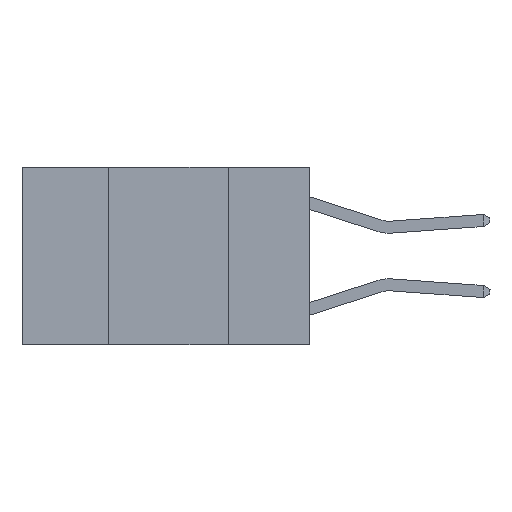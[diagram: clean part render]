
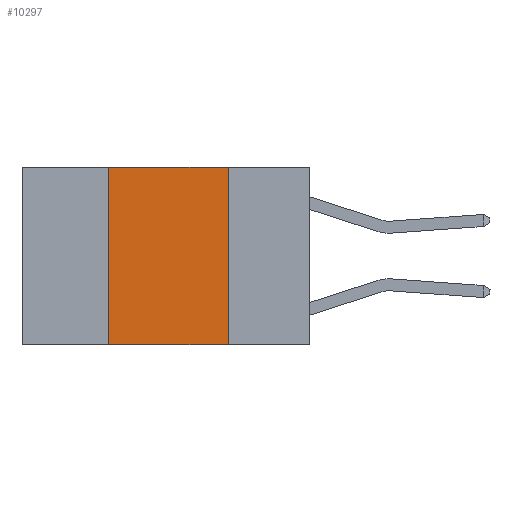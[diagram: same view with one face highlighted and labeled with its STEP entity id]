
A CAD part, left-side view. The second image highlights one B-rep face of the part: STEP entity #10297.
In plain terms, the highlighted planar face has unit normal (-1, 0, 0).
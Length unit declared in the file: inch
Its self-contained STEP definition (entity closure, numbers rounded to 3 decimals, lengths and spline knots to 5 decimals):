
#68 = DIRECTION ( 'NONE',  ( 0., 0., 1. ) ) ;
#74 = CARTESIAN_POINT ( 'NONE',  ( 0., 0.6, 0. ) ) ;
#545 = EDGE_CURVE ( 'NONE', #13243, #10573, #12109, .T. ) ;
#1654 = CARTESIAN_POINT ( 'NONE',  ( 0., 0.42, -0.37 ) ) ;
#2096 = LINE ( 'NONE', #6562, #13497 ) ;
#3424 = DIRECTION ( 'NONE',  ( 1., 0., 0. ) ) ;
#3793 = EDGE_CURVE ( 'NONE', #12015, #11036, #11168, .T. ) ;
#4370 = EDGE_CURVE ( 'NONE', #10573, #12015, #13056, .T. ) ;
#4399 = DIRECTION ( 'NONE',  ( 0., -1., 0. ) ) ;
#4626 = CARTESIAN_POINT ( 'NONE',  ( 0., 0.17, -0.37 ) ) ;
#4745 = FACE_OUTER_BOUND ( 'NONE', #12834, .T. ) ;
#5888 = VECTOR ( 'NONE', #68, 39.37008 ) ;
#6309 = CARTESIAN_POINT ( 'NONE',  ( 0., 0.17, 0. ) ) ;
#6562 = CARTESIAN_POINT ( 'NONE',  ( 0., 0.6, -0.37 ) ) ;
#7415 = DIRECTION ( 'NONE',  ( 0., 0., -1. ) ) ;
#7454 = ORIENTED_EDGE ( 'NONE', *, *, #4370, .F. ) ;
#7796 = ORIENTED_EDGE ( 'NONE', *, *, #12215, .T. ) ;
#8273 = DIRECTION ( 'NONE',  ( 0., -1., 0. ) ) ;
#8881 = CARTESIAN_POINT ( 'NONE',  ( 0., 0.42, 0. ) ) ;
#10297 = ADVANCED_FACE ( 'NONE', ( #4745 ), #13325, .F. ) ;
#10413 = ORIENTED_EDGE ( 'NONE', *, *, #545, .F. ) ;
#10573 = VERTEX_POINT ( 'NONE', #13809 ) ;
#11036 = VERTEX_POINT ( 'NONE', #4626 ) ;
#11160 = DIRECTION ( 'NONE',  ( 0., 0., -1. ) ) ;
#11168 = LINE ( 'NONE', #6309, #13763 ) ;
#11779 = AXIS2_PLACEMENT_3D ( 'NONE', #74, #3424, #11160 ) ;
#12015 = VERTEX_POINT ( 'NONE', #12948 ) ;
#12109 = LINE ( 'NONE', #8881, #5888 ) ;
#12215 = EDGE_CURVE ( 'NONE', #13243, #11036, #2096, .T. ) ;
#12363 = VECTOR ( 'NONE', #8273, 39.37008 ) ;
#12684 = CARTESIAN_POINT ( 'NONE',  ( 0., 0.6, 0. ) ) ;
#12834 = EDGE_LOOP ( 'NONE', ( #12990, #7454, #10413, #7796 ) ) ;
#12948 = CARTESIAN_POINT ( 'NONE',  ( 0., 0.17, 0. ) ) ;
#12990 = ORIENTED_EDGE ( 'NONE', *, *, #3793, .F. ) ;
#13056 = LINE ( 'NONE', #12684, #12363 ) ;
#13243 = VERTEX_POINT ( 'NONE', #1654 ) ;
#13325 = PLANE ( 'NONE',  #11779 ) ;
#13497 = VECTOR ( 'NONE', #4399, 39.37008 ) ;
#13763 = VECTOR ( 'NONE', #7415, 39.37008 ) ;
#13809 = CARTESIAN_POINT ( 'NONE',  ( 0., 0.42, 0. ) ) ;
